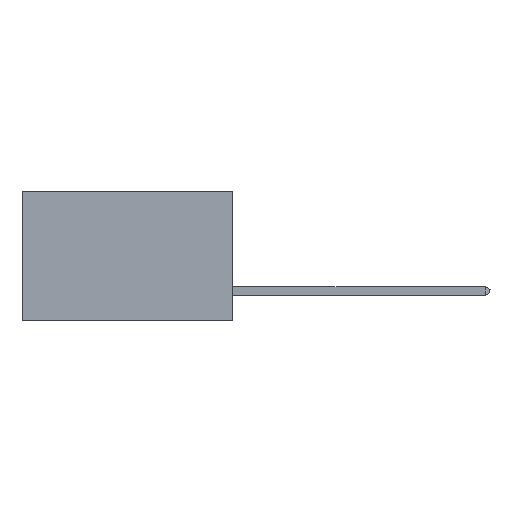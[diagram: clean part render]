
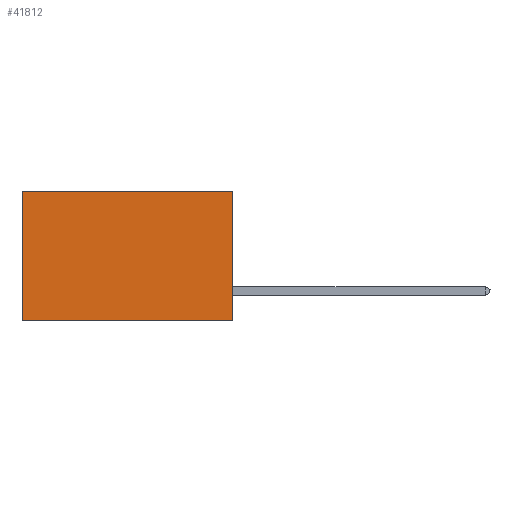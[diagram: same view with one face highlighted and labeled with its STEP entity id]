
A CAD part, left-side view. The second image highlights one B-rep face of the part: STEP entity #41812.
In plain terms, the highlighted planar face has unit normal (-1, 0, 0).
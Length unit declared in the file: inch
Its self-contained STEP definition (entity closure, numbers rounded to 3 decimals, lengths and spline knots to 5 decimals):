
#881 = LINE ( 'NONE', #39046, #13811 ) ;
#1689 = ORIENTED_EDGE ( 'NONE', *, *, #17079, .T. ) ;
#1903 = VERTEX_POINT ( 'NONE', #4038 ) ;
#2895 = EDGE_CURVE ( 'NONE', #34234, #14952, #24471, .T. ) ;
#4038 = CARTESIAN_POINT ( 'NONE',  ( 0.2875, 0.6, 0. ) ) ;
#8557 = VECTOR ( 'NONE', #13822, 39.37008 ) ;
#8589 = LINE ( 'NONE', #22216, #34571 ) ;
#9636 = LINE ( 'NONE', #34553, #8557 ) ;
#9668 = CARTESIAN_POINT ( 'NONE',  ( 0.2875, 0., 0. ) ) ;
#11940 = FACE_OUTER_BOUND ( 'NONE', #35142, .T. ) ;
#11953 = DIRECTION ( 'NONE',  ( 0., 1., 0. ) ) ;
#13603 = CARTESIAN_POINT ( 'NONE',  ( 0.2875, 0., 0. ) ) ;
#13811 = VECTOR ( 'NONE', #18004, 39.37008 ) ;
#13822 = DIRECTION ( 'NONE',  ( 0., 0., -1. ) ) ;
#14952 = VERTEX_POINT ( 'NONE', #24735 ) ;
#15051 = DIRECTION ( 'NONE',  ( 1., 0., 0. ) ) ;
#16390 = VERTEX_POINT ( 'NONE', #42231 ) ;
#17079 = EDGE_CURVE ( 'NONE', #1903, #16390, #9636, .T. ) ;
#18004 = DIRECTION ( 'NONE',  ( 0., 1., 0. ) ) ;
#22216 = CARTESIAN_POINT ( 'NONE',  ( 0.2875, 0., -0.37 ) ) ;
#24471 = LINE ( 'NONE', #9668, #28823 ) ;
#24735 = CARTESIAN_POINT ( 'NONE',  ( 0.2875, 0., -0.37 ) ) ;
#27205 = DIRECTION ( 'NONE',  ( 0., 0., -1. ) ) ;
#28612 = ORIENTED_EDGE ( 'NONE', *, *, #31143, .F. ) ;
#28823 = VECTOR ( 'NONE', #27205, 39.37008 ) ;
#28999 = CARTESIAN_POINT ( 'NONE',  ( 0.2875, 0., 0. ) ) ;
#31143 = EDGE_CURVE ( 'NONE', #14952, #16390, #8589, .T. ) ;
#31423 = ORIENTED_EDGE ( 'NONE', *, *, #2895, .F. ) ;
#32445 = DIRECTION ( 'NONE',  ( 0., 0., -1. ) ) ;
#32694 = EDGE_CURVE ( 'NONE', #34234, #1903, #881, .T. ) ;
#34234 = VERTEX_POINT ( 'NONE', #13603 ) ;
#34553 = CARTESIAN_POINT ( 'NONE',  ( 0.2875, 0.6, 0. ) ) ;
#34571 = VECTOR ( 'NONE', #11953, 39.37008 ) ;
#35142 = EDGE_LOOP ( 'NONE', ( #1689, #28612, #31423, #41540 ) ) ;
#36205 = PLANE ( 'NONE',  #40881 ) ;
#39046 = CARTESIAN_POINT ( 'NONE',  ( 0.2875, 0., 0. ) ) ;
#40881 = AXIS2_PLACEMENT_3D ( 'NONE', #28999, #15051, #32445 ) ;
#41540 = ORIENTED_EDGE ( 'NONE', *, *, #32694, .T. ) ;
#41812 = ADVANCED_FACE ( 'NONE', ( #11940 ), #36205, .F. ) ;
#42231 = CARTESIAN_POINT ( 'NONE',  ( 0.2875, 0.6, -0.37 ) ) ;
